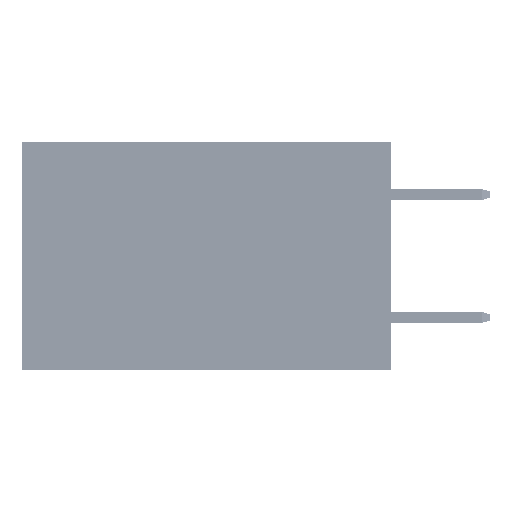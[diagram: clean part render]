
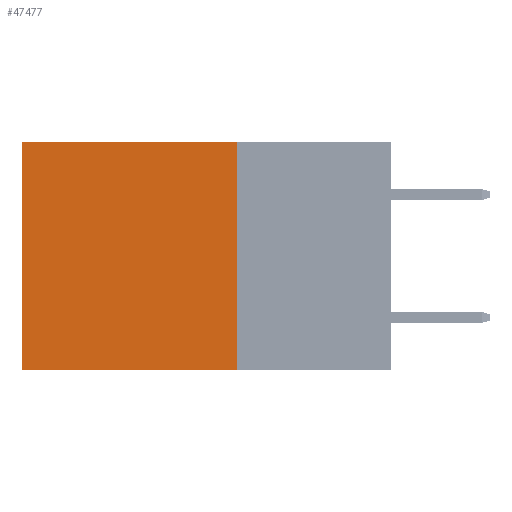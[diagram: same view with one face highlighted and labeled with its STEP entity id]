
A CAD part, left-side view. The second image highlights one B-rep face of the part: STEP entity #47477.
In plain terms, the highlighted planar face has unit normal (-1, 0, 0).
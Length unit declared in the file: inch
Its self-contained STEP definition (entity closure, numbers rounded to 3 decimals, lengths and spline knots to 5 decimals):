
#1214 = LINE ( 'NONE', #35196, #9885 ) ;
#7256 = CARTESIAN_POINT ( 'NONE',  ( 0.2875, 0.25, -0.37 ) ) ;
#9162 = CARTESIAN_POINT ( 'NONE',  ( 0.2875, 0.25, 0. ) ) ;
#9885 = VECTOR ( 'NONE', #19376, 39.37008 ) ;
#10696 = DIRECTION ( 'NONE',  ( 0., 0., -1. ) ) ;
#12954 = PLANE ( 'NONE',  #18475 ) ;
#13136 = DIRECTION ( 'NONE',  ( 0., 0., -1. ) ) ;
#14751 = LINE ( 'NONE', #18968, #38186 ) ;
#16862 = VERTEX_POINT ( 'NONE', #35277 ) ;
#18125 = EDGE_CURVE ( 'NONE', #28745, #16862, #32578, .T. ) ;
#18475 = AXIS2_PLACEMENT_3D ( 'NONE', #9162, #40560, #44515 ) ;
#18968 = CARTESIAN_POINT ( 'NONE',  ( 0.2875, 0.25, 0. ) ) ;
#19376 = DIRECTION ( 'NONE',  ( 0., 1., 0. ) ) ;
#23155 = FACE_OUTER_BOUND ( 'NONE', #27983, .T. ) ;
#23754 = ORIENTED_EDGE ( 'NONE', *, *, #31289, .T. ) ;
#26750 = DIRECTION ( 'NONE',  ( 0., 1., 0. ) ) ;
#27513 = EDGE_CURVE ( 'NONE', #33729, #16862, #42455, .T. ) ;
#27983 = EDGE_LOOP ( 'NONE', ( #28315, #50822, #45847, #23754 ) ) ;
#28315 = ORIENTED_EDGE ( 'NONE', *, *, #27513, .T. ) ;
#28745 = VERTEX_POINT ( 'NONE', #43718 ) ;
#28875 = VECTOR ( 'NONE', #13136, 39.37008 ) ;
#30189 = VERTEX_POINT ( 'NONE', #31163 ) ;
#31163 = CARTESIAN_POINT ( 'NONE',  ( 0.2875, 0.25, 0. ) ) ;
#31289 = EDGE_CURVE ( 'NONE', #30189, #33729, #1214, .T. ) ;
#31324 = VECTOR ( 'NONE', #26750, 39.37008 ) ;
#31959 = EDGE_CURVE ( 'NONE', #30189, #28745, #14751, .T. ) ;
#32578 = LINE ( 'NONE', #7256, #31324 ) ;
#33729 = VERTEX_POINT ( 'NONE', #34375 ) ;
#34375 = CARTESIAN_POINT ( 'NONE',  ( 0.2875, 0.6, 0. ) ) ;
#35196 = CARTESIAN_POINT ( 'NONE',  ( 0.2875, 0.25, 0. ) ) ;
#35277 = CARTESIAN_POINT ( 'NONE',  ( 0.2875, 0.6, -0.37 ) ) ;
#38186 = VECTOR ( 'NONE', #10696, 39.37008 ) ;
#40560 = DIRECTION ( 'NONE',  ( 1., 0., 0. ) ) ;
#42455 = LINE ( 'NONE', #48347, #28875 ) ;
#43718 = CARTESIAN_POINT ( 'NONE',  ( 0.2875, 0.25, -0.37 ) ) ;
#44515 = DIRECTION ( 'NONE',  ( 0., 0., -1. ) ) ;
#45847 = ORIENTED_EDGE ( 'NONE', *, *, #31959, .F. ) ;
#47477 = ADVANCED_FACE ( 'NONE', ( #23155 ), #12954, .F. ) ;
#48347 = CARTESIAN_POINT ( 'NONE',  ( 0.2875, 0.6, 0. ) ) ;
#50822 = ORIENTED_EDGE ( 'NONE', *, *, #18125, .F. ) ;
